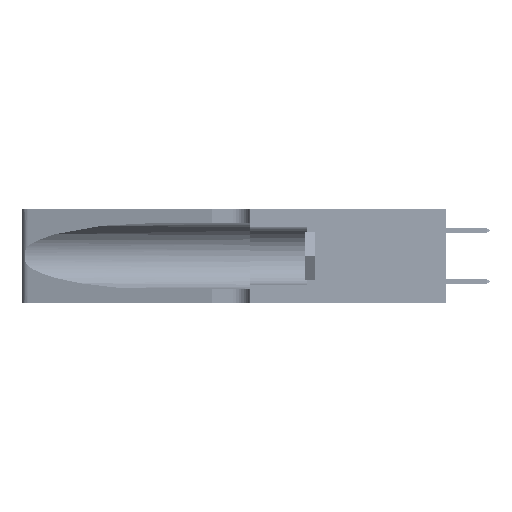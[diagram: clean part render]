
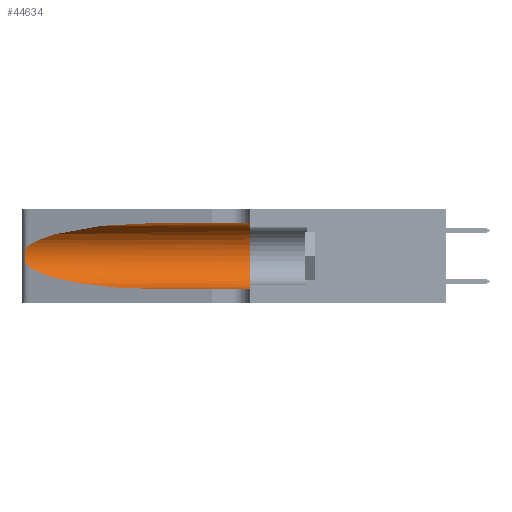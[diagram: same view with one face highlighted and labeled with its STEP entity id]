
A CAD part, left-side view. The second image highlights one B-rep face of the part: STEP entity #44634.
In plain terms, the highlighted cylindrical face has radius 3.308 mm (diameter 6.617 mm), a partial arc.
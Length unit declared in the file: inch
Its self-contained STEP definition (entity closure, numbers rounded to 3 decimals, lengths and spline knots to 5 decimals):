
#2094 = AXIS2_PLACEMENT_3D ( 'NONE', #2184, #40285, #44471 ) ;
#2184 = CARTESIAN_POINT ( 'NONE',  ( 0.1305, 1.61858, 0.185 ) ) ;
#2970 = CARTESIAN_POINT ( 'NONE',  ( 0.26018, 1.23835, 0.19895 ) ) ;
#3026 = ORIENTED_EDGE ( 'NONE', *, *, #17330, .F. ) ;
#3031 = EDGE_CURVE ( 'NONE', #15733, #42769, #45967, .T. ) ;
#3137 = CARTESIAN_POINT ( 'NONE',  ( 0.25789, 1.23486, 0.15765 ) ) ;
#3296 = CARTESIAN_POINT ( 'NONE',  ( 0.25555, 1.22994, 0.2215 ) ) ;
#3581 = CARTESIAN_POINT ( 'NONE',  ( 0.1305, 0.72297, 0.31525 ) ) ;
#6981 = CARTESIAN_POINT ( 'NONE',  ( 0.25639, 1.23186, 0.15144 ) ) ;
#7193 = DIRECTION ( 'NONE',  ( 0., 1., 0. ) ) ;
#7495 = VECTOR ( 'NONE', #25278, 39.37008 ) ;
#7838 = ORIENTED_EDGE ( 'NONE', *, *, #13696, .T. ) ;
#8115 = CARTESIAN_POINT ( 'NONE',  ( 0.25487, 1.22718, 0.22369 ) ) ;
#8465 = ORIENTED_EDGE ( 'NONE', *, *, #3031, .T. ) ;
#8940 = CARTESIAN_POINT ( 'NONE',  ( 0.1305, 0.35, 0.31525 ) ) ;
#10681 = CARTESIAN_POINT ( 'NONE',  ( 0.25555, 1.22993, 0.14849 ) ) ;
#11009 = CARTESIAN_POINT ( 'NONE',  ( 0.26075, 1.23896, 0.178 ) ) ;
#11162 = AXIS2_PLACEMENT_3D ( 'NONE', #18617, #7193, #49329 ) ;
#11328 = VERTEX_POINT ( 'NONE', #3581 ) ;
#11355 = CARTESIAN_POINT ( 'NONE',  ( 0.25787, 1.23484, 0.2124 ) ) ;
#12323 = LINE ( 'NONE', #25750, #7495 ) ;
#13696 = EDGE_CURVE ( 'NONE', #27303, #20466, #14814, .T. ) ;
#14814 = B_SPLINE_CURVE_WITH_KNOTS ( 'NONE', 3,
 ( #37527, #3296, #14895, #11355, #49136, #2970, #49290, #11009, #34168, #41380, #3137, #6981, #10681, #29971 ),
 .UNSPECIFIED., .F., .F.,
 ( 4, 2, 2, 2, 2, 2, 4 ),
 ( 0., 0.00027, 0.00053, 0.00107, 0.0016, 0.00187, 0.00214 ),
 .UNSPECIFIED. ) ;
#14895 = CARTESIAN_POINT ( 'NONE',  ( 0.25639, 1.23184, 0.21858 ) ) ;
#15299 = EDGE_CURVE ( 'NONE', #11328, #27303, #45892, .T. ) ;
#15605 = CARTESIAN_POINT ( 'NONE',  ( 0.2373, 1.15595, 0.08982 ) ) ;
#15733 = VERTEX_POINT ( 'NONE', #28195 ) ;
#17177 = CARTESIAN_POINT ( 'NONE',  ( 0.1305, 0.35, 0.05475 ) ) ;
#17330 = EDGE_CURVE ( 'NONE', #11328, #46767, #12323, .T. ) ;
#18121 = CARTESIAN_POINT ( 'NONE',  ( 0.25487, 1.22718, 0.14631 ) ) ;
#18617 = CARTESIAN_POINT ( 'NONE',  ( 0.1305, 0.35, 0.185 ) ) ;
#20466 = VERTEX_POINT ( 'NONE', #18121 ) ;
#22357 = CARTESIAN_POINT ( 'NONE',  ( 0.18966, 0.96281, 0.31525 ) ) ;
#23334 = CARTESIAN_POINT ( 'NONE',  ( 0.1305, 0.72297, 0.05475 ) ) ;
#23566 = EDGE_CURVE ( 'NONE', #46767, #42769, #29527, .T. ) ;
#25278 = DIRECTION ( 'NONE',  ( 0., -1., 0. ) ) ;
#25659 = EDGE_LOOP ( 'NONE', ( #29857, #7838, #36492, #8465, #31654, #3026 ) ) ;
#25750 = CARTESIAN_POINT ( 'NONE',  ( 0.1305, 1.61858, 0.31525 ) ) ;
#26457 = DIRECTION ( 'NONE',  ( 0., -1., 0. ) ) ;
#26990 = CARTESIAN_POINT ( 'NONE',  ( 0.25487, 1.22718, 0.14631 ) ) ;
#27303 = VERTEX_POINT ( 'NONE', #8115 ) ;
#28138 = CYLINDRICAL_SURFACE ( 'NONE', #2094, 0.13025 ) ;
#28195 = CARTESIAN_POINT ( 'NONE',  ( 0.1305, 0.72297, 0.05475 ) ) ;
#29527 = CIRCLE ( 'NONE', #11162, 0.13025 ) ;
#29665 = CARTESIAN_POINT ( 'NONE',  ( 0.1305, 1.61858, 0.05475 ) ) ;
#29857 = ORIENTED_EDGE ( 'NONE', *, *, #15299, .T. ) ;
#29910 = CARTESIAN_POINT ( 'NONE',  ( 0.1305, 0.72297, 0.31525 ) ) ;
#29971 = CARTESIAN_POINT ( 'NONE',  ( 0.25487, 1.22718, 0.14631 ) ) ;
#31654 = ORIENTED_EDGE ( 'NONE', *, *, #23566, .F. ) ;
#34168 = CARTESIAN_POINT ( 'NONE',  ( 0.26017, 1.23833, 0.17102 ) ) ;
#34757 = FACE_OUTER_BOUND ( 'NONE', #25659, .T. ) ;
#36492 = ORIENTED_EDGE ( 'NONE', *, *, #47296, .T. ) ;
#37527 = CARTESIAN_POINT ( 'NONE',  ( 0.25487, 1.22718, 0.22369 ) ) ;
#39930 = VECTOR ( 'NONE', #26457, 39.37008 ) ;
#40285 = DIRECTION ( 'NONE',  ( 0., -1., 0. ) ) ;
#41380 = CARTESIAN_POINT ( 'NONE',  ( 0.25856, 1.23593, 0.16098 ) ) ;
#41646 = CARTESIAN_POINT ( 'NONE',  ( 0.2373, 1.15595, 0.28018 ) ) ;
#42152 = CARTESIAN_POINT ( 'NONE',  ( 0.25487, 1.22718, 0.22369 ) ) ;
#42769 = VERTEX_POINT ( 'NONE', #17177 ) ;
#44351 =( BOUNDED_CURVE ( )  B_SPLINE_CURVE ( 3, ( #26990, #15605, #46315, #23334 ),
 .UNSPECIFIED., .F., .F. ) 
 B_SPLINE_CURVE_WITH_KNOTS ( ( 4, 4 ),
 ( 3.44316, 4.71239 ),
 .UNSPECIFIED. ) 
 CURVE ( )  GEOMETRIC_REPRESENTATION_ITEM ( )  RATIONAL_B_SPLINE_CURVE ( ( 1., 0.87, 0.87, 1. ) ) 
 REPRESENTATION_ITEM ( '' )  );
#44471 = DIRECTION ( 'NONE',  ( 0., 0., -1. ) ) ;
#44634 = ADVANCED_FACE ( 'NONE', ( #34757 ), #28138, .F. ) ;
#45892 =( BOUNDED_CURVE ( )  B_SPLINE_CURVE ( 3, ( #29910, #22357, #41646, #42152 ),
 .UNSPECIFIED., .F., .T. ) 
 B_SPLINE_CURVE_WITH_KNOTS ( ( 4, 4 ),
 ( 1.5708, 2.84003 ),
 .UNSPECIFIED. ) 
 CURVE ( )  GEOMETRIC_REPRESENTATION_ITEM ( )  RATIONAL_B_SPLINE_CURVE ( ( 1., 0.87, 0.87, 1. ) ) 
 REPRESENTATION_ITEM ( '' )  );
#45967 = LINE ( 'NONE', #29665, #39930 ) ;
#46315 = CARTESIAN_POINT ( 'NONE',  ( 0.18966, 0.96281, 0.05475 ) ) ;
#46767 = VERTEX_POINT ( 'NONE', #8940 ) ;
#47296 = EDGE_CURVE ( 'NONE', #20466, #15733, #44351, .T. ) ;
#49136 = CARTESIAN_POINT ( 'NONE',  ( 0.25854, 1.2359, 0.20912 ) ) ;
#49290 = CARTESIAN_POINT ( 'NONE',  ( 0.26075, 1.23896, 0.19203 ) ) ;
#49329 = DIRECTION ( 'NONE',  ( 0., 0., 1. ) ) ;
